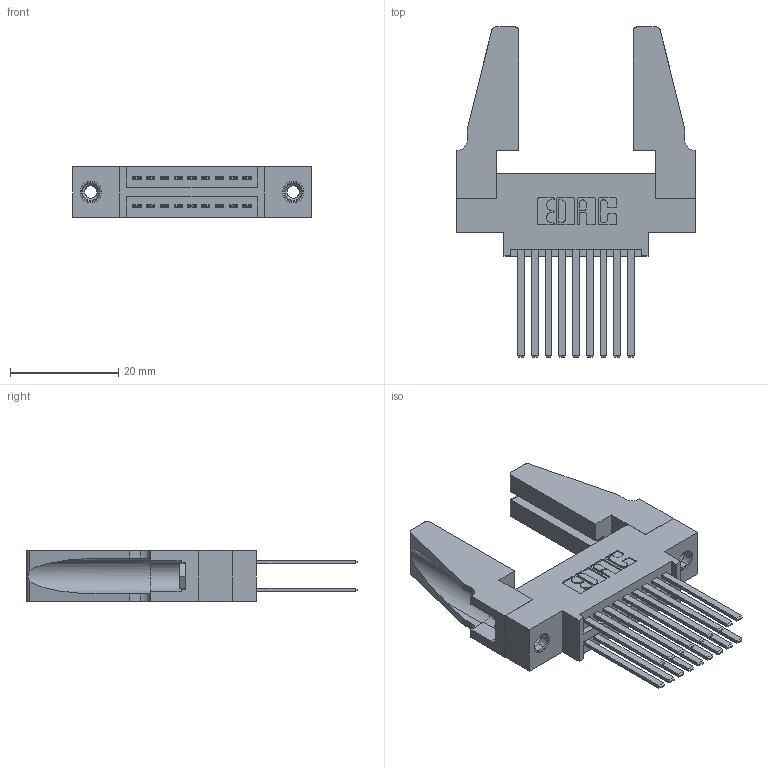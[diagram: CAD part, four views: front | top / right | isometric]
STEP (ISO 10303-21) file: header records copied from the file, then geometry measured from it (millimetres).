
FILE_DESCRIPTION (( 'STEP AP203' ), '1' );
FILE_NAME ('345-018-544-888.STEP', '2019-10-27T06:39:25', ( '' ), ( '' ), 'SwSTEP 2.0', 'SolidWorks 2016', '' );
FILE_SCHEMA (( 'CONFIG_CONTROL_DESIGN' ));
Length unit declared in the file: inch
Products named in the file (5): 345-220-078_345-220-088; 345-250-001_345-250-001-102; 345 Part_0.170 Offset - 0.156 Dia-TH; 345-018-544-888; 345-292-001_345-293-144
Assembly tree (23 placements, depth 2):
  345-018-544-888
    345 Part_0.170 Offset - 0.156 Dia-TH
    345-292-001_345-293-144  x18
    345-250-001_345-250-001-102  x2
    345-220-078_345-220-088  x2
Bounding box: 44.09 x 61.14 x 9.4 mm (x, y, z)
Volume: 7368.4 mm3; surface area: 9450.1 mm2
Topology: 23 solids, 23 shells, 1046 faces, 3025 edges, 1982 vertices
Faces by surface type: plane 678, cylinder 352, cone 12, torus 4
Entity records: 13600 total; most frequent: CARTESIAN_POINT 2306, ORIENTED_EDGE 2200, DIRECTION 2076, EDGE_CURVE 1100, VECTOR 894, LINE 894, VERTEX_POINT 726, AXIS2_PLACEMENT_3D 591
